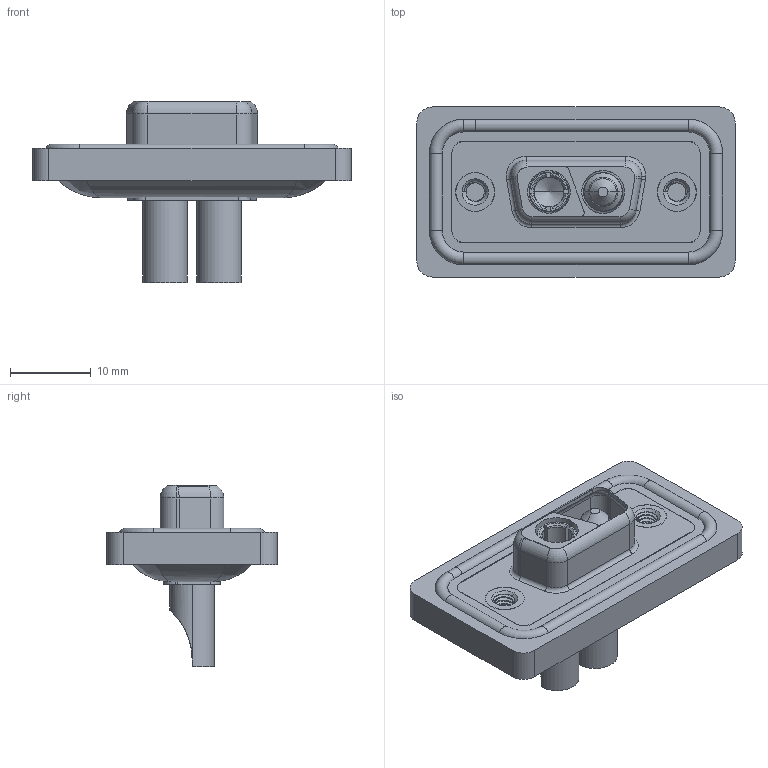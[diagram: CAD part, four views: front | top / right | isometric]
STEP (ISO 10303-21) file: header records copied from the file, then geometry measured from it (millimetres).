
FILE_DESCRIPTION (( 'STEP AP203' ), '1' );
FILE_NAME ('628W2WK2322-4NA.STEP', '2024-03-22T13:11:17', ( '' ), ( '' ), 'SwSTEP 2.0', 'SolidWorks 2023', '' );
FILE_SCHEMA (( 'CONFIG_CONTROL_DESIGN' ));
Length unit declared in the file: millimetre
Products named in the file (8): 628Combo Shell Front_09 Contacts; 628Combo Shell Rear_09 Contacts; 628W2WK2322-4NA; Power Pin_40A SC; 628Combo Waterproof Housing_09 Contacts; 628Combo Housing_2WK2; Power Socket_40A SC; 628Combo Threaded Rivet_A
Assembly tree (8 placements, depth 2):
  628W2WK2322-4NA
    628Combo Housing_2WK2
    628Combo Waterproof Housing_09 Contacts
    628Combo Shell Front_09 Contacts
    628Combo Shell Rear_09 Contacts
    628Combo Threaded Rivet_A  x2
    Power Socket_40A SC
    Power Pin_40A SC
Bounding box: 39.5 x 21.1 x 22.45 mm (x, y, z)
Volume: 4684.4 mm3; surface area: 7621 mm2
Topology: 11 solids, 11 shells, 504 faces, 1246 edges, 775 vertices
Faces by surface type: cylinder 235, plane 148, torus 77, cone 32, bspline 12
Entity records: 17209 total; most frequent: CARTESIAN_POINT 5108, DIRECTION 2461, ORIENTED_EDGE 2308, EDGE_CURVE 1154, AXIS2_PLACEMENT_3D 978, VERTEX_POINT 725, EDGE_LOOP 515, VECTOR 505
